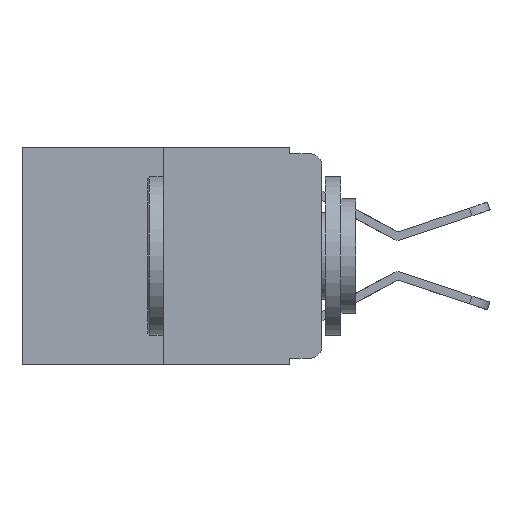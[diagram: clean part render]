
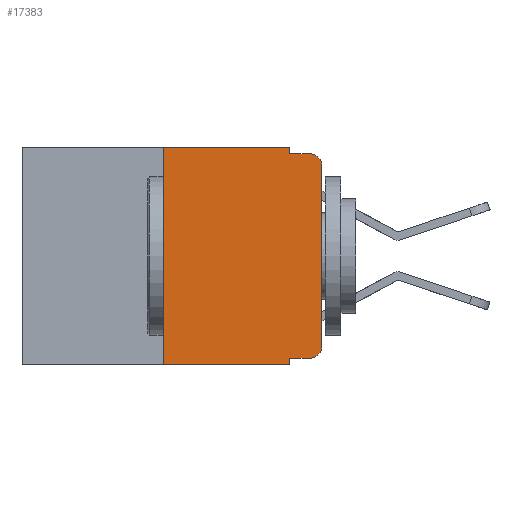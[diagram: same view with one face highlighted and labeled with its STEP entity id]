
A CAD part, left-side view. The second image highlights one B-rep face of the part: STEP entity #17383.
In plain terms, the highlighted planar face has unit normal (-1, 0, 0).
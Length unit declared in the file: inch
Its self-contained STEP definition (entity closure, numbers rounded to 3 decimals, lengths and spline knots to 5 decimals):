
#274 = ORIENTED_EDGE ( 'NONE', *, *, #20563, .T. ) ;
#427 = VERTEX_POINT ( 'NONE', #24666 ) ;
#467 = DIRECTION ( 'NONE',  ( -1., 0., 0. ) ) ;
#525 = LINE ( 'NONE', #16171, #16338 ) ;
#723 = CARTESIAN_POINT ( 'NONE',  ( 0., 0.051, -0.343 ) ) ;
#1385 = CARTESIAN_POINT ( 'NONE',  ( 0., 0.051, -0.333 ) ) ;
#1823 = VERTEX_POINT ( 'NONE', #25424 ) ;
#2347 = VERTEX_POINT ( 'NONE', #13774 ) ;
#2600 = ORIENTED_EDGE ( 'NONE', *, *, #23233, .T. ) ;
#3409 = CARTESIAN_POINT ( 'NONE',  ( 0., 0.02, -0.333 ) ) ;
#3496 = DIRECTION ( 'NONE',  ( 0., -1., 0. ) ) ;
#3893 = DIRECTION ( 'NONE',  ( 0., 0., -1. ) ) ;
#4697 = VECTOR ( 'NONE', #7290, 39.37008 ) ;
#4867 = ORIENTED_EDGE ( 'NONE', *, *, #5089, .F. ) ;
#5089 = EDGE_CURVE ( 'NONE', #1823, #2347, #14717, .T. ) ;
#5276 = VECTOR ( 'NONE', #23761, 39.37008 ) ;
#6179 = VERTEX_POINT ( 'NONE', #17358 ) ;
#6792 = ORIENTED_EDGE ( 'NONE', *, *, #10954, .T. ) ;
#7062 = EDGE_CURVE ( 'NONE', #2347, #427, #525, .T. ) ;
#7290 = DIRECTION ( 'NONE',  ( 0., 0., 1. ) ) ;
#7523 = EDGE_CURVE ( 'NONE', #427, #10807, #10708, .T. ) ;
#8263 = CARTESIAN_POINT ( 'NONE',  ( 0., 0.02, -0.03 ) ) ;
#8618 = LINE ( 'NONE', #24031, #18738 ) ;
#8903 = VECTOR ( 'NONE', #3893, 39.37008 ) ;
#9629 = CARTESIAN_POINT ( 'NONE',  ( 0., 0.051, 0. ) ) ;
#10197 = LINE ( 'NONE', #12017, #8903 ) ;
#10240 = CARTESIAN_POINT ( 'NONE',  ( 0., 0., -0.03 ) ) ;
#10292 = AXIS2_PLACEMENT_3D ( 'NONE', #12773, #467, #14779 ) ;
#10305 = DIRECTION ( 'NONE',  ( 0., 0., -1. ) ) ;
#10340 = CARTESIAN_POINT ( 'NONE',  ( 0., 0.473, 0. ) ) ;
#10708 = LINE ( 'NONE', #9629, #5276 ) ;
#10807 = VERTEX_POINT ( 'NONE', #15597 ) ;
#10954 = EDGE_CURVE ( 'NONE', #1823, #16975, #22018, .T. ) ;
#11353 = CARTESIAN_POINT ( 'NONE',  ( 0., 0., -0.313 ) ) ;
#11534 = VERTEX_POINT ( 'NONE', #18294 ) ;
#11983 = DIRECTION ( 'NONE',  ( 0., -1., 0. ) ) ;
#12005 = VERTEX_POINT ( 'NONE', #10240 ) ;
#12017 = CARTESIAN_POINT ( 'NONE',  ( 0., 0.051, 0. ) ) ;
#12386 = DIRECTION ( 'NONE',  ( 0., 0., -1. ) ) ;
#12546 = EDGE_LOOP ( 'NONE', ( #274, #13137, #23861, #14392, #25108, #4867, #6792, #17533, #2600, #13463 ) ) ;
#12773 = CARTESIAN_POINT ( 'NONE',  ( 0., 0.02, -0.313 ) ) ;
#13137 = ORIENTED_EDGE ( 'NONE', *, *, #19748, .T. ) ;
#13463 = ORIENTED_EDGE ( 'NONE', *, *, #17823, .T. ) ;
#13774 = CARTESIAN_POINT ( 'NONE',  ( 0., 0.25, 0. ) ) ;
#14077 = CIRCLE ( 'NONE', #16698, 0.02 ) ;
#14313 = EDGE_CURVE ( 'NONE', #10807, #11534, #8618, .T. ) ;
#14392 = ORIENTED_EDGE ( 'NONE', *, *, #7523, .F. ) ;
#14652 = DIRECTION ( 'NONE',  ( 0., 0., 1. ) ) ;
#14717 = LINE ( 'NONE', #22654, #24815 ) ;
#14779 = DIRECTION ( 'NONE',  ( 0., 0., -1. ) ) ;
#15102 = FACE_OUTER_BOUND ( 'NONE', #12546, .T. ) ;
#15597 = CARTESIAN_POINT ( 'NONE',  ( 0., 0.051, -0.01 ) ) ;
#16171 = CARTESIAN_POINT ( 'NONE',  ( 0., 0.473, 0. ) ) ;
#16306 = PLANE ( 'NONE',  #18060 ) ;
#16338 = VECTOR ( 'NONE', #18214, 39.37008 ) ;
#16488 = VERTEX_POINT ( 'NONE', #3409 ) ;
#16698 = AXIS2_PLACEMENT_3D ( 'NONE', #8263, #22371, #10305 ) ;
#16975 = VERTEX_POINT ( 'NONE', #723 ) ;
#17238 = VECTOR ( 'NONE', #11983, 39.37008 ) ;
#17358 = CARTESIAN_POINT ( 'NONE',  ( 0., 0.051, -0.333 ) ) ;
#17383 = ADVANCED_FACE ( 'NONE', ( #15102 ), #16306, .F. ) ;
#17533 = ORIENTED_EDGE ( 'NONE', *, *, #24572, .F. ) ;
#17593 = CIRCLE ( 'NONE', #10292, 0.02 ) ;
#17823 = EDGE_CURVE ( 'NONE', #16488, #23727, #17593, .T. ) ;
#18060 = AXIS2_PLACEMENT_3D ( 'NONE', #10340, #24448, #12386 ) ;
#18214 = DIRECTION ( 'NONE',  ( 0., -1., 0. ) ) ;
#18294 = CARTESIAN_POINT ( 'NONE',  ( 0., 0.02, -0.01 ) ) ;
#18458 = VECTOR ( 'NONE', #3496, 39.37008 ) ;
#18738 = VECTOR ( 'NONE', #25990, 39.37008 ) ;
#19114 = LINE ( 'NONE', #1385, #18458 ) ;
#19748 = EDGE_CURVE ( 'NONE', #12005, #11534, #14077, .T. ) ;
#20563 = EDGE_CURVE ( 'NONE', #23727, #12005, #20845, .T. ) ;
#20845 = LINE ( 'NONE', #21340, #4697 ) ;
#21340 = CARTESIAN_POINT ( 'NONE',  ( 0., 0., 0. ) ) ;
#22018 = LINE ( 'NONE', #26026, #17238 ) ;
#22371 = DIRECTION ( 'NONE',  ( -1., 0., 0. ) ) ;
#22654 = CARTESIAN_POINT ( 'NONE',  ( 0., 0.25, 0. ) ) ;
#23233 = EDGE_CURVE ( 'NONE', #6179, #16488, #19114, .T. ) ;
#23727 = VERTEX_POINT ( 'NONE', #11353 ) ;
#23761 = DIRECTION ( 'NONE',  ( 0., 0., -1. ) ) ;
#23861 = ORIENTED_EDGE ( 'NONE', *, *, #14313, .F. ) ;
#24031 = CARTESIAN_POINT ( 'NONE',  ( 0., 0.051, -0.01 ) ) ;
#24448 = DIRECTION ( 'NONE',  ( 1., 0., 0. ) ) ;
#24572 = EDGE_CURVE ( 'NONE', #6179, #16975, #10197, .T. ) ;
#24666 = CARTESIAN_POINT ( 'NONE',  ( 0., 0.051, 0. ) ) ;
#24815 = VECTOR ( 'NONE', #14652, 39.37008 ) ;
#25108 = ORIENTED_EDGE ( 'NONE', *, *, #7062, .F. ) ;
#25424 = CARTESIAN_POINT ( 'NONE',  ( 0., 0.25, -0.343 ) ) ;
#25990 = DIRECTION ( 'NONE',  ( 0., -1., 0. ) ) ;
#26026 = CARTESIAN_POINT ( 'NONE',  ( 0., 0.473, -0.343 ) ) ;
